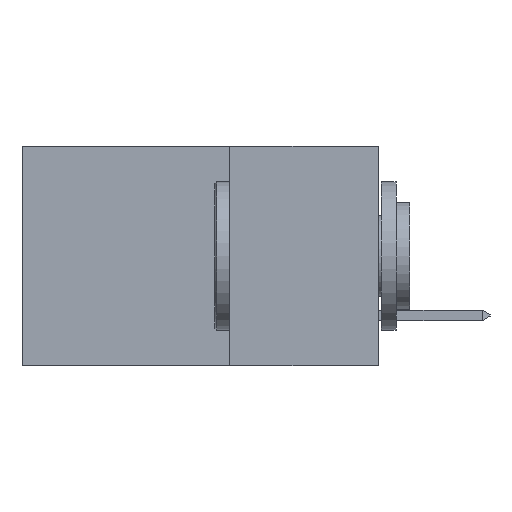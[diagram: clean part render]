
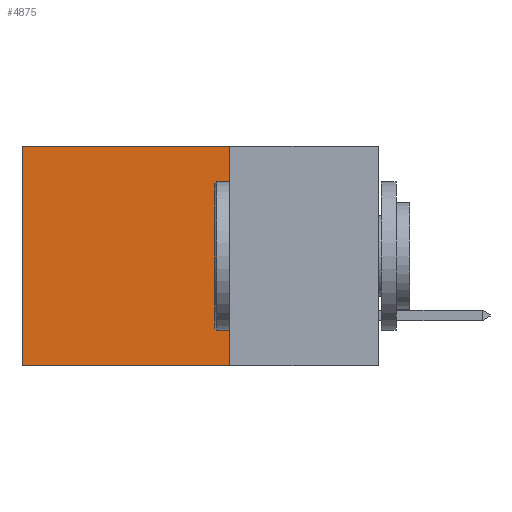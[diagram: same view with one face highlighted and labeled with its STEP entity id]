
A CAD part, left-side view. The second image highlights one B-rep face of the part: STEP entity #4875.
In plain terms, the highlighted planar face has unit normal (-1, 0, 0).
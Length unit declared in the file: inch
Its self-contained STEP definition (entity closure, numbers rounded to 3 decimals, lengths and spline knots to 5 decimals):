
#292 = VECTOR ( 'NONE', #14725, 39.37008 ) ;
#375 = CARTESIAN_POINT ( 'NONE',  ( 0.2615, 0.25, -0.37 ) ) ;
#786 = CARTESIAN_POINT ( 'NONE',  ( 0.2615, 0.25, 0. ) ) ;
#2229 = EDGE_CURVE ( 'NONE', #4710, #12412, #4165, .T. ) ;
#4165 = LINE ( 'NONE', #6960, #13750 ) ;
#4710 = VERTEX_POINT ( 'NONE', #786 ) ;
#4875 = ADVANCED_FACE ( 'NONE', ( #6097 ), #15728, .F. ) ;
#5079 = VERTEX_POINT ( 'NONE', #14264 ) ;
#5518 = ORIENTED_EDGE ( 'NONE', *, *, #2229, .F. ) ;
#6097 = FACE_OUTER_BOUND ( 'NONE', #6541, .T. ) ;
#6264 = DIRECTION ( 'NONE',  ( 0., 0., -1. ) ) ;
#6541 = EDGE_LOOP ( 'NONE', ( #7469, #13139, #5518, #10009 ) ) ;
#6658 = DIRECTION ( 'NONE',  ( 0., 1., 0. ) ) ;
#6960 = CARTESIAN_POINT ( 'NONE',  ( 0.2615, 0.25, -0.37 ) ) ;
#7469 = ORIENTED_EDGE ( 'NONE', *, *, #12421, .T. ) ;
#8313 = CARTESIAN_POINT ( 'NONE',  ( 0.2615, 0.6, -0.37 ) ) ;
#8636 = EDGE_CURVE ( 'NONE', #4710, #15307, #8662, .T. ) ;
#8662 = LINE ( 'NONE', #9552, #14685 ) ;
#9006 = AXIS2_PLACEMENT_3D ( 'NONE', #15677, #15638, #15623 ) ;
#9552 = CARTESIAN_POINT ( 'NONE',  ( 0.2615, 0.25, 0. ) ) ;
#10009 = ORIENTED_EDGE ( 'NONE', *, *, #8636, .T. ) ;
#10565 = CARTESIAN_POINT ( 'NONE',  ( 0.2615, 0.6, 0. ) ) ;
#10762 = LINE ( 'NONE', #8313, #292 ) ;
#11102 = EDGE_CURVE ( 'NONE', #12412, #5079, #15788, .T. ) ;
#12412 = VERTEX_POINT ( 'NONE', #375 ) ;
#12421 = EDGE_CURVE ( 'NONE', #15307, #5079, #10762, .T. ) ;
#13139 = ORIENTED_EDGE ( 'NONE', *, *, #11102, .F. ) ;
#13421 = DIRECTION ( 'NONE',  ( 0., 1., 0. ) ) ;
#13750 = VECTOR ( 'NONE', #6264, 39.37008 ) ;
#14264 = CARTESIAN_POINT ( 'NONE',  ( 0.2615, 0.6, -0.37 ) ) ;
#14394 = CARTESIAN_POINT ( 'NONE',  ( 0.2615, 0.25, -0.37 ) ) ;
#14685 = VECTOR ( 'NONE', #13421, 39.37008 ) ;
#14725 = DIRECTION ( 'NONE',  ( 0., 0., -1. ) ) ;
#15307 = VERTEX_POINT ( 'NONE', #10565 ) ;
#15623 = DIRECTION ( 'NONE',  ( 0., 0., -1. ) ) ;
#15638 = DIRECTION ( 'NONE',  ( 1., 0., 0. ) ) ;
#15677 = CARTESIAN_POINT ( 'NONE',  ( 0.2615, 0.25, -0.37 ) ) ;
#15728 = PLANE ( 'NONE',  #9006 ) ;
#15788 = LINE ( 'NONE', #14394, #16183 ) ;
#16183 = VECTOR ( 'NONE', #6658, 39.37008 ) ;
